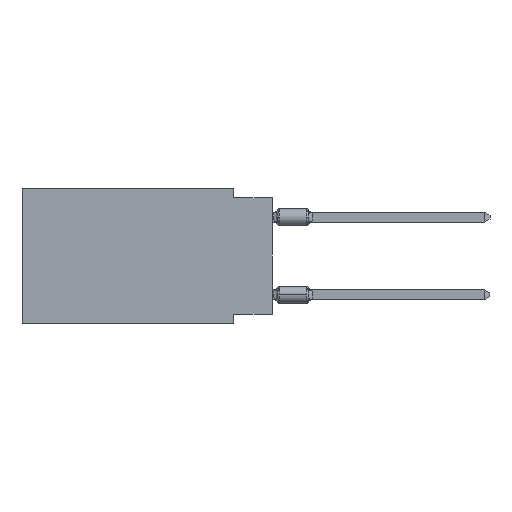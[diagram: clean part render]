
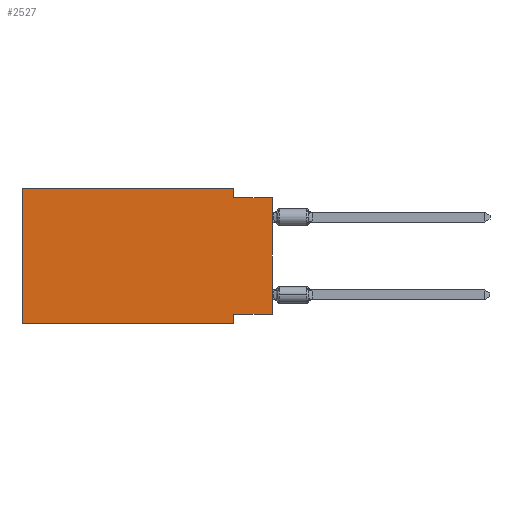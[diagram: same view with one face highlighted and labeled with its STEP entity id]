
A CAD part, left-side view. The second image highlights one B-rep face of the part: STEP entity #2527.
In plain terms, the highlighted planar face has unit normal (-1, 0, 0).
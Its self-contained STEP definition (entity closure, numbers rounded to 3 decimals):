
#69 = CARTESIAN_POINT ( 'NONE',  ( 0., 16.383, -8.89 ) ) ;
#940 = VECTOR ( 'NONE', #9332, 1000. ) ;
#1600 = VERTEX_POINT ( 'NONE', #13003 ) ;
#1750 = CARTESIAN_POINT ( 'NONE',  ( 0., 0., -8.255 ) ) ;
#1923 = ORIENTED_EDGE ( 'NONE', *, *, #2449, .T. ) ;
#1946 = VECTOR ( 'NONE', #10825, 1000. ) ;
#2124 = LINE ( 'NONE', #6326, #12901 ) ;
#2213 = CARTESIAN_POINT ( 'NONE',  ( 0., 0., -8.255 ) ) ;
#2279 = LINE ( 'NONE', #69, #1946 ) ;
#2414 = FACE_OUTER_BOUND ( 'NONE', #10536, .T. ) ;
#2449 = EDGE_CURVE ( 'NONE', #3099, #1600, #2279, .T. ) ;
#2527 = ADVANCED_FACE ( 'NONE', ( #2414 ), #6484, .F. ) ;
#2608 = AXIS2_PLACEMENT_3D ( 'NONE', #7659, #11859, #4408 ) ;
#2654 = ORIENTED_EDGE ( 'NONE', *, *, #7909, .F. ) ;
#2695 = CARTESIAN_POINT ( 'NONE',  ( 0., 0., 0. ) ) ;
#2838 = VERTEX_POINT ( 'NONE', #11501 ) ;
#2999 = VECTOR ( 'NONE', #5569, 1000. ) ;
#3099 = VERTEX_POINT ( 'NONE', #6803 ) ;
#3460 = VECTOR ( 'NONE', #12372, 1000. ) ;
#3653 = DIRECTION ( 'NONE',  ( 0., 0., 1. ) ) ;
#4052 = ORIENTED_EDGE ( 'NONE', *, *, #6125, .F. ) ;
#4317 = EDGE_CURVE ( 'NONE', #2838, #9523, #2124, .T. ) ;
#4408 = DIRECTION ( 'NONE',  ( 0., 0., -1. ) ) ;
#5094 = VERTEX_POINT ( 'NONE', #10561 ) ;
#5489 = EDGE_CURVE ( 'NONE', #5094, #1600, #9922, .T. ) ;
#5569 = DIRECTION ( 'NONE',  ( 0., 0., -1. ) ) ;
#5612 = DIRECTION ( 'NONE',  ( 0., -1., 0. ) ) ;
#6095 = LINE ( 'NONE', #8172, #3460 ) ;
#6125 = EDGE_CURVE ( 'NONE', #11888, #2838, #6095, .T. ) ;
#6326 = CARTESIAN_POINT ( 'NONE',  ( 0., 2.54, 0. ) ) ;
#6484 = PLANE ( 'NONE',  #2608 ) ;
#6562 = CARTESIAN_POINT ( 'NONE',  ( 0., 0., -0.635 ) ) ;
#6803 = CARTESIAN_POINT ( 'NONE',  ( 0., 16.383, -8.89 ) ) ;
#7182 = ORIENTED_EDGE ( 'NONE', *, *, #11297, .F. ) ;
#7278 = VECTOR ( 'NONE', #5612, 1000. ) ;
#7650 = ORIENTED_EDGE ( 'NONE', *, *, #4317, .F. ) ;
#7659 = CARTESIAN_POINT ( 'NONE',  ( 0., 16.383, 0. ) ) ;
#7715 = CARTESIAN_POINT ( 'NONE',  ( 0., 16.383, 0. ) ) ;
#7867 = CARTESIAN_POINT ( 'NONE',  ( 0., 16.383, 0. ) ) ;
#7908 = VECTOR ( 'NONE', #11101, 1000. ) ;
#7909 = EDGE_CURVE ( 'NONE', #3099, #11888, #11163, .T. ) ;
#7930 = EDGE_CURVE ( 'NONE', #11512, #10625, #12133, .T. ) ;
#8172 = CARTESIAN_POINT ( 'NONE',  ( 0., 16.383, 0. ) ) ;
#8919 = CARTESIAN_POINT ( 'NONE',  ( 0., 0., -0.635 ) ) ;
#9267 = ORIENTED_EDGE ( 'NONE', *, *, #12506, .F. ) ;
#9332 = DIRECTION ( 'NONE',  ( 0., 1., 0. ) ) ;
#9523 = VERTEX_POINT ( 'NONE', #12592 ) ;
#9922 = LINE ( 'NONE', #10749, #2999 ) ;
#10329 = VECTOR ( 'NONE', #3653, 1000. ) ;
#10534 = DIRECTION ( 'NONE',  ( 0., 0., -1. ) ) ;
#10536 = EDGE_LOOP ( 'NONE', ( #13619, #7182, #7650, #4052, #2654, #1923, #11240, #9267 ) ) ;
#10561 = CARTESIAN_POINT ( 'NONE',  ( 0., 2.54, -8.255 ) ) ;
#10625 = VERTEX_POINT ( 'NONE', #6562 ) ;
#10749 = CARTESIAN_POINT ( 'NONE',  ( 0., 2.54, -8.89 ) ) ;
#10800 = LINE ( 'NONE', #8919, #7278 ) ;
#10825 = DIRECTION ( 'NONE',  ( 0., -1., 0. ) ) ;
#11101 = DIRECTION ( 'NONE',  ( 0., 0., 1. ) ) ;
#11163 = LINE ( 'NONE', #7867, #10329 ) ;
#11240 = ORIENTED_EDGE ( 'NONE', *, *, #5489, .F. ) ;
#11297 = EDGE_CURVE ( 'NONE', #9523, #10625, #10800, .T. ) ;
#11501 = CARTESIAN_POINT ( 'NONE',  ( 0., 2.54, 0. ) ) ;
#11512 = VERTEX_POINT ( 'NONE', #2213 ) ;
#11859 = DIRECTION ( 'NONE',  ( 1., 0., 0. ) ) ;
#11888 = VERTEX_POINT ( 'NONE', #7715 ) ;
#12133 = LINE ( 'NONE', #2695, #7908 ) ;
#12295 = LINE ( 'NONE', #1750, #940 ) ;
#12372 = DIRECTION ( 'NONE',  ( 0., -1., 0. ) ) ;
#12506 = EDGE_CURVE ( 'NONE', #11512, #5094, #12295, .T. ) ;
#12592 = CARTESIAN_POINT ( 'NONE',  ( 0., 2.54, -0.635 ) ) ;
#12901 = VECTOR ( 'NONE', #10534, 1000. ) ;
#13003 = CARTESIAN_POINT ( 'NONE',  ( 0., 2.54, -8.89 ) ) ;
#13619 = ORIENTED_EDGE ( 'NONE', *, *, #7930, .T. ) ;
